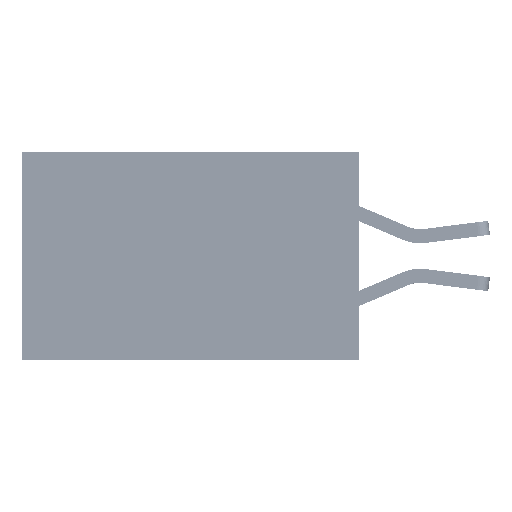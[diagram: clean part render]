
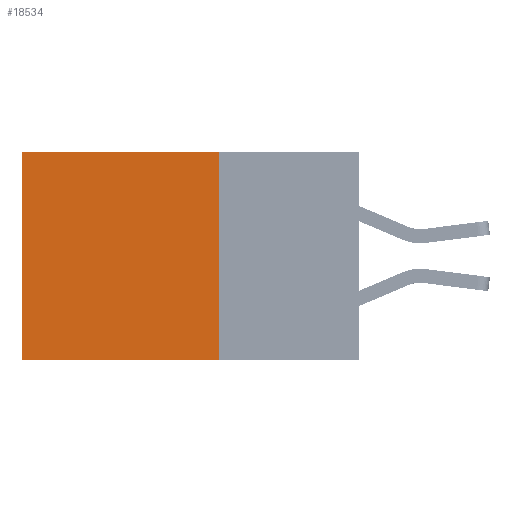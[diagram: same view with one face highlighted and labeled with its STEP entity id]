
A CAD part, left-side view. The second image highlights one B-rep face of the part: STEP entity #18534.
In plain terms, the highlighted planar face has unit normal (-1, 0, 0).
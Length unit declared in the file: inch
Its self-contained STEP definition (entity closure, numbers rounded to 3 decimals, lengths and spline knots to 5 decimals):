
#821 = CARTESIAN_POINT ( 'NONE',  ( 0.2875, 0.6, -0.37 ) ) ;
#1083 = CARTESIAN_POINT ( 'NONE',  ( 0.2875, 0.25, 0. ) ) ;
#2016 = VERTEX_POINT ( 'NONE', #32645 ) ;
#2438 = EDGE_CURVE ( 'NONE', #6497, #16750, #29383, .T. ) ;
#3746 = CARTESIAN_POINT ( 'NONE',  ( 0.2875, 0.6, 0. ) ) ;
#4304 = EDGE_CURVE ( 'NONE', #2016, #6497, #21656, .T. ) ;
#5847 = EDGE_LOOP ( 'NONE', ( #18968, #18443, #13257, #24055 ) ) ;
#6283 = DIRECTION ( 'NONE',  ( 1., 0., 0. ) ) ;
#6497 = VERTEX_POINT ( 'NONE', #13171 ) ;
#7687 = DIRECTION ( 'NONE',  ( 0., 1., 0. ) ) ;
#9429 = CARTESIAN_POINT ( 'NONE',  ( 0.2875, 0.25, 0. ) ) ;
#11552 = VECTOR ( 'NONE', #7687, 39.37008 ) ;
#12596 = FACE_OUTER_BOUND ( 'NONE', #5847, .T. ) ;
#13171 = CARTESIAN_POINT ( 'NONE',  ( 0.2875, 0.6, 0. ) ) ;
#13257 = ORIENTED_EDGE ( 'NONE', *, *, #37123, .F. ) ;
#16750 = VERTEX_POINT ( 'NONE', #821 ) ;
#18443 = ORIENTED_EDGE ( 'NONE', *, *, #23842, .F. ) ;
#18534 = ADVANCED_FACE ( 'NONE', ( #12596 ), #25431, .F. ) ;
#18968 = ORIENTED_EDGE ( 'NONE', *, *, #2438, .T. ) ;
#19109 = DIRECTION ( 'NONE',  ( 0., 0., -1. ) ) ;
#21656 = LINE ( 'NONE', #34461, #31165 ) ;
#21987 = CARTESIAN_POINT ( 'NONE',  ( 0.2875, 0.25, -0.37 ) ) ;
#23506 = DIRECTION ( 'NONE',  ( 0., 0., -1. ) ) ;
#23842 = EDGE_CURVE ( 'NONE', #38546, #16750, #29549, .T. ) ;
#23978 = DIRECTION ( 'NONE',  ( 0., 1., 0. ) ) ;
#24055 = ORIENTED_EDGE ( 'NONE', *, *, #4304, .T. ) ;
#25431 = PLANE ( 'NONE',  #39964 ) ;
#29383 = LINE ( 'NONE', #3746, #38797 ) ;
#29549 = LINE ( 'NONE', #36070, #11552 ) ;
#31165 = VECTOR ( 'NONE', #23978, 39.37008 ) ;
#32430 = LINE ( 'NONE', #1083, #37175 ) ;
#32645 = CARTESIAN_POINT ( 'NONE',  ( 0.2875, 0.25, 0. ) ) ;
#33046 = DIRECTION ( 'NONE',  ( 0., 0., -1. ) ) ;
#34461 = CARTESIAN_POINT ( 'NONE',  ( 0.2875, 0.25, 0. ) ) ;
#36070 = CARTESIAN_POINT ( 'NONE',  ( 0.2875, 0.25, -0.37 ) ) ;
#37123 = EDGE_CURVE ( 'NONE', #2016, #38546, #32430, .T. ) ;
#37175 = VECTOR ( 'NONE', #33046, 39.37008 ) ;
#38546 = VERTEX_POINT ( 'NONE', #21987 ) ;
#38797 = VECTOR ( 'NONE', #23506, 39.37008 ) ;
#39964 = AXIS2_PLACEMENT_3D ( 'NONE', #9429, #6283, #19109 ) ;
